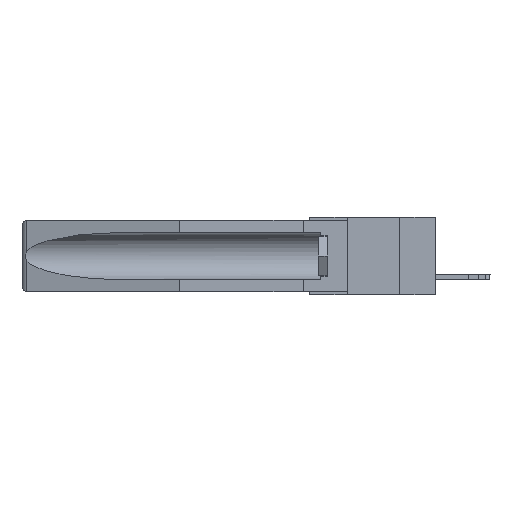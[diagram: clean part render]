
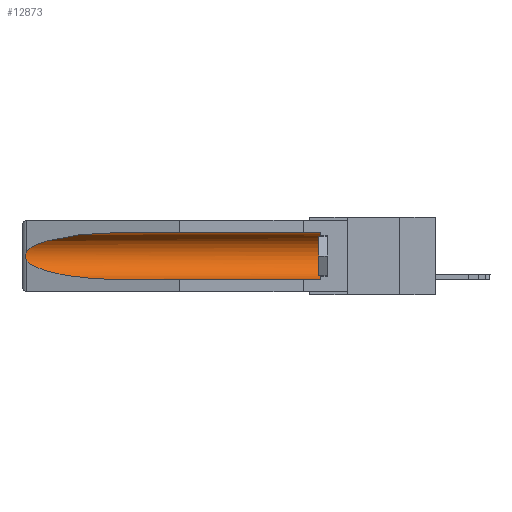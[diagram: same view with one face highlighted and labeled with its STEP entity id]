
A CAD part, left-side view. The second image highlights one B-rep face of the part: STEP entity #12873.
In plain terms, the highlighted cylindrical face has radius 2.857 mm (diameter 5.715 mm), a partial arc.
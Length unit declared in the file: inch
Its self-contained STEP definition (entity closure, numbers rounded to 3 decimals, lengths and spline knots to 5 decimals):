
#111 = DIRECTION ( 'NONE',  ( 0., 1., 0. ) ) ;
#222 = CARTESIAN_POINT ( 'NONE',  ( 0.26537, 1.52718, -0.19328 ) ) ;
#1527 = ORIENTED_EDGE ( 'NONE', *, *, #17285, .T. ) ;
#1660 = VERTEX_POINT ( 'NONE', #2737 ) ;
#1670 = CARTESIAN_POINT ( 'NONE',  ( 0.155, 1.07973, -0.284 ) ) ;
#1817 = CARTESIAN_POINT ( 'NONE',  ( 0.26655, 1.53094, -0.18657 ) ) ;
#1997 = CARTESIAN_POINT ( 'NONE',  ( 0.155, -0.30754, -0.059 ) ) ;
#2193 = DIRECTION ( 'NONE',  ( 0., 1., 0. ) ) ;
#2718 = DIRECTION ( 'NONE',  ( 0., 0., 1. ) ) ;
#2737 = CARTESIAN_POINT ( 'NONE',  ( 0.155, 1.07973, -0.284 ) ) ;
#2755 = EDGE_CURVE ( 'NONE', #20990, #3477, #7094, .T. ) ;
#3461 = CARTESIAN_POINT ( 'NONE',  ( 0.2673, 1.5327, -0.16383 ) ) ;
#3477 = VERTEX_POINT ( 'NONE', #9068 ) ;
#3778 = EDGE_CURVE ( 'NONE', #12136, #20990, #13304, .T. ) ;
#4088 = CARTESIAN_POINT ( 'NONE',  ( 0.155, -0.30754, -0.1715 ) ) ;
#4785 = CARTESIAN_POINT ( 'NONE',  ( 0.26537, 1.52718, -0.14972 ) ) ;
#5208 = CARTESIAN_POINT ( 'NONE',  ( 0.155, 0.126, -0.284 ) ) ;
#5498 = EDGE_CURVE ( 'NONE', #13641, #12136, #21539, .T. ) ;
#5790 = EDGE_LOOP ( 'NONE', ( #14190, #21148, #20398, #6794, #1527, #11100 ) ) ;
#6009 = CARTESIAN_POINT ( 'NONE',  ( 0.155, 0.126, -0.1715 ) ) ;
#6594 = CARTESIAN_POINT ( 'NONE',  ( 0.26537, 1.52718, -0.14972 ) ) ;
#6794 = ORIENTED_EDGE ( 'NONE', *, *, #17158, .F. ) ;
#6904 = CARTESIAN_POINT ( 'NONE',  ( 0.26537, 1.52718, -0.14972 ) ) ;
#7094 = B_SPLINE_CURVE_WITH_KNOTS ( 'NONE', 3,
 ( #6904, #7123, #11998, #3461, #20567, #10422, #15337, #1817, #13688, #222 ),
 .UNSPECIFIED., .F., .F.,
 ( 4, 2, 2, 2, 4 ),
 ( 0., 0.00029, 0.00058, 0.00087, 0.00117 ),
 .UNSPECIFIED. ) ;
#7123 = CARTESIAN_POINT ( 'NONE',  ( 0.26597, 1.52961, -0.15275 ) ) ;
#8976 = VECTOR ( 'NONE', #2193, 39.37008 ) ;
#9068 = CARTESIAN_POINT ( 'NONE',  ( 0.26537, 1.52718, -0.19328 ) ) ;
#10422 = CARTESIAN_POINT ( 'NONE',  ( 0.2675, 1.53308, -0.17534 ) ) ;
#10818 = CARTESIAN_POINT ( 'NONE',  ( 0.155, 0.126, -0.059 ) ) ;
#11100 = ORIENTED_EDGE ( 'NONE', *, *, #5498, .T. ) ;
#11132 =( BOUNDED_CURVE ( )  B_SPLINE_CURVE ( 3, ( #15192, #11332, #16936, #1670 ),
 .UNSPECIFIED., .F., .F. ) 
 B_SPLINE_CURVE_WITH_KNOTS ( ( 4, 4 ),
 ( 0.1948, 1.5708 ),
 .UNSPECIFIED. ) 
 CURVE ( )  GEOMETRIC_REPRESENTATION_ITEM ( )  RATIONAL_B_SPLINE_CURVE ( ( 1., 0.848, 0.848, 1. ) ) 
 REPRESENTATION_ITEM ( '' )  );
#11332 = CARTESIAN_POINT ( 'NONE',  ( 0.25451, 1.48313, -0.24835 ) ) ;
#11594 = CARTESIAN_POINT ( 'NONE',  ( 0.25451, 1.48313, -0.09465 ) ) ;
#11693 = VECTOR ( 'NONE', #111, 39.37008 ) ;
#11998 = CARTESIAN_POINT ( 'NONE',  ( 0.26654, 1.53092, -0.15636 ) ) ;
#12136 = VERTEX_POINT ( 'NONE', #13038 ) ;
#12604 = AXIS2_PLACEMENT_3D ( 'NONE', #6009, #17956, #2718 ) ;
#12873 = ADVANCED_FACE ( 'NONE', ( #14102 ), #16457, .F. ) ;
#13038 = CARTESIAN_POINT ( 'NONE',  ( 0.155, 1.07973, -0.059 ) ) ;
#13304 =( BOUNDED_CURVE ( )  B_SPLINE_CURVE ( 3, ( #14774, #16732, #11594, #4785 ),
 .UNSPECIFIED., .F., .F. ) 
 B_SPLINE_CURVE_WITH_KNOTS ( ( 4, 4 ),
 ( 4.71239, 6.08839 ),
 .UNSPECIFIED. ) 
 CURVE ( )  GEOMETRIC_REPRESENTATION_ITEM ( )  RATIONAL_B_SPLINE_CURVE ( ( 1., 0.848, 0.848, 1. ) ) 
 REPRESENTATION_ITEM ( '' )  );
#13641 = VERTEX_POINT ( 'NONE', #10818 ) ;
#13688 = CARTESIAN_POINT ( 'NONE',  ( 0.26597, 1.5296, -0.19026 ) ) ;
#14102 = FACE_OUTER_BOUND ( 'NONE', #5790, .T. ) ;
#14190 = ORIENTED_EDGE ( 'NONE', *, *, #3778, .T. ) ;
#14774 = CARTESIAN_POINT ( 'NONE',  ( 0.155, 1.07973, -0.059 ) ) ;
#15192 = CARTESIAN_POINT ( 'NONE',  ( 0.26537, 1.52718, -0.19328 ) ) ;
#15337 = CARTESIAN_POINT ( 'NONE',  ( 0.2673, 1.53269, -0.17917 ) ) ;
#15547 = AXIS2_PLACEMENT_3D ( 'NONE', #4088, #20940, #17451 ) ;
#15641 = LINE ( 'NONE', #17518, #8976 ) ;
#16457 = CYLINDRICAL_SURFACE ( 'NONE', #15547, 0.1125 ) ;
#16732 = CARTESIAN_POINT ( 'NONE',  ( 0.21114, 1.30732, -0.059 ) ) ;
#16904 = EDGE_CURVE ( 'NONE', #3477, #1660, #11132, .T. ) ;
#16936 = CARTESIAN_POINT ( 'NONE',  ( 0.21114, 1.30732, -0.284 ) ) ;
#17158 = EDGE_CURVE ( 'NONE', #20536, #1660, #15641, .T. ) ;
#17285 = EDGE_CURVE ( 'NONE', #20536, #13641, #21234, .T. ) ;
#17451 = DIRECTION ( 'NONE',  ( 0., 0., 1. ) ) ;
#17518 = CARTESIAN_POINT ( 'NONE',  ( 0.155, -0.30754, -0.284 ) ) ;
#17956 = DIRECTION ( 'NONE',  ( 0., -1., 0. ) ) ;
#20398 = ORIENTED_EDGE ( 'NONE', *, *, #16904, .T. ) ;
#20536 = VERTEX_POINT ( 'NONE', #5208 ) ;
#20567 = CARTESIAN_POINT ( 'NONE',  ( 0.2675, 1.53308, -0.16763 ) ) ;
#20940 = DIRECTION ( 'NONE',  ( 0., 1., 0. ) ) ;
#20990 = VERTEX_POINT ( 'NONE', #6594 ) ;
#21148 = ORIENTED_EDGE ( 'NONE', *, *, #2755, .T. ) ;
#21234 = CIRCLE ( 'NONE', #12604, 0.1125 ) ;
#21539 = LINE ( 'NONE', #1997, #11693 ) ;
